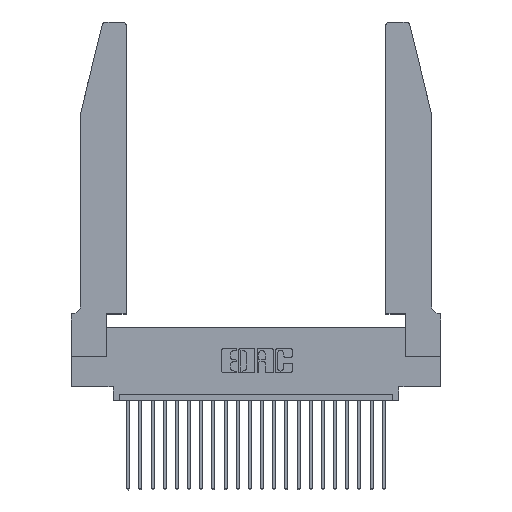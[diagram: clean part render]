
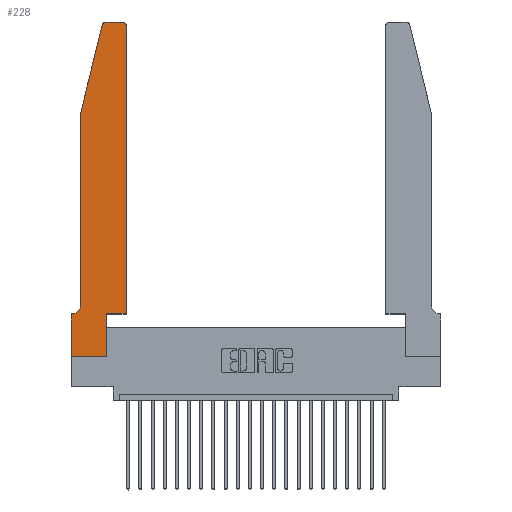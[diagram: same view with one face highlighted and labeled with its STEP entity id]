
A CAD part, top view. The second image highlights one B-rep face of the part: STEP entity #228.
In plain terms, the highlighted planar face has unit normal (0, 0, 1).
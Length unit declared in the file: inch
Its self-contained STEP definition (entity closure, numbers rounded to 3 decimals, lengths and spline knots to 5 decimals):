
#208 = DIRECTION ( 'NONE',  ( 0., -1., 0. ) ) ;
#228 = ADVANCED_FACE ( 'NONE', ( #15772 ), #24019, .T. ) ;
#949 = VECTOR ( 'NONE', #1038, 39.37008 ) ;
#1038 = DIRECTION ( 'NONE',  ( -0.239, -0.971, 0. ) ) ;
#1377 = VERTEX_POINT ( 'NONE', #22624 ) ;
#1398 = ORIENTED_EDGE ( 'NONE', *, *, #16703, .T. ) ;
#1642 = CARTESIAN_POINT ( 'NONE',  ( 0., 0.35, 0.37 ) ) ;
#1769 = VERTEX_POINT ( 'NONE', #23635 ) ;
#1843 = CARTESIAN_POINT ( 'NONE',  ( 0., 0.35, 0.37 ) ) ;
#1872 = ORIENTED_EDGE ( 'NONE', *, *, #16879, .T. ) ;
#2104 = LINE ( 'NONE', #21125, #12880 ) ;
#2142 = CARTESIAN_POINT ( 'NONE',  ( 0., 0., 0.37 ) ) ;
#2615 = VERTEX_POINT ( 'NONE', #24074 ) ;
#2848 = DIRECTION ( 'NONE',  ( 0., 0., -1. ) ) ;
#3400 = EDGE_CURVE ( 'NONE', #4514, #14230, #17943, .T. ) ;
#3630 = ORIENTED_EDGE ( 'NONE', *, *, #4726, .T. ) ;
#3846 = VERTEX_POINT ( 'NONE', #20107 ) ;
#3853 = EDGE_CURVE ( 'NONE', #1769, #8784, #18219, .T. ) ;
#4328 = DIRECTION ( 'NONE',  ( -1., 0., 0. ) ) ;
#4514 = VERTEX_POINT ( 'NONE', #21830 ) ;
#4726 = EDGE_CURVE ( 'NONE', #20221, #5148, #13159, .T. ) ;
#4738 = DIRECTION ( 'NONE',  ( -1., 0., 0. ) ) ;
#4908 = EDGE_CURVE ( 'NONE', #15444, #2615, #2104, .T. ) ;
#4972 = DIRECTION ( 'NONE',  ( 0., 1., 0. ) ) ;
#5030 = EDGE_CURVE ( 'NONE', #3846, #13183, #15221, .T. ) ;
#5148 = VERTEX_POINT ( 'NONE', #2142 ) ;
#5470 = EDGE_LOOP ( 'NONE', ( #20709, #20847, #14493, #20641, #1872, #21702, #3630, #16234, #9642, #24148, #1398, #8935 ) ) ;
#5584 = EDGE_CURVE ( 'NONE', #5148, #11150, #21610, .T. ) ;
#5921 = CARTESIAN_POINT ( 'NONE',  ( 0.0755, 0.35, 0.37 ) ) ;
#6894 = LINE ( 'NONE', #17451, #19441 ) ;
#7106 = VECTOR ( 'NONE', #10693, 39.37008 ) ;
#7161 = CIRCLE ( 'NONE', #9581, 0.07 ) ;
#8303 = CARTESIAN_POINT ( 'NONE',  ( 0.0755, 2., 0.37 ) ) ;
#8549 = CARTESIAN_POINT ( 'NONE',  ( 0.0755, 2., 0.37 ) ) ;
#8784 = VERTEX_POINT ( 'NONE', #10356 ) ;
#8935 = ORIENTED_EDGE ( 'NONE', *, *, #3853, .T. ) ;
#9190 = EDGE_CURVE ( 'NONE', #1377, #20221, #10885, .T. ) ;
#9581 = AXIS2_PLACEMENT_3D ( 'NONE', #14099, #2848, #4738 ) ;
#9642 = ORIENTED_EDGE ( 'NONE', *, *, #22647, .T. ) ;
#9996 = LINE ( 'NONE', #10611, #7106 ) ;
#10356 = CARTESIAN_POINT ( 'NONE',  ( 0.4205, 2.75, 0.37 ) ) ;
#10611 = CARTESIAN_POINT ( 'NONE',  ( 0.2865, 0.35, 0.37 ) ) ;
#10693 = DIRECTION ( 'NONE',  ( 0., 1., 0. ) ) ;
#10829 = VECTOR ( 'NONE', #208, 39.37008 ) ;
#10885 = LINE ( 'NONE', #5921, #21707 ) ;
#11150 = VERTEX_POINT ( 'NONE', #20236 ) ;
#11836 = DIRECTION ( 'NONE',  ( 0., -1., 0. ) ) ;
#12509 = DIRECTION ( 'NONE',  ( 1., 0., 0. ) ) ;
#12837 = DIRECTION ( 'NONE',  ( 1., 0., 0. ) ) ;
#12880 = VECTOR ( 'NONE', #11836, 39.37008 ) ;
#13157 = AXIS2_PLACEMENT_3D ( 'NONE', #13678, #17201, #17374 ) ;
#13159 = LINE ( 'NONE', #13223, #10829 ) ;
#13183 = VERTEX_POINT ( 'NONE', #17450 ) ;
#13223 = CARTESIAN_POINT ( 'NONE',  ( 0., 0., 0.37 ) ) ;
#13304 = AXIS2_PLACEMENT_3D ( 'NONE', #16375, #23688, #12509 ) ;
#13678 = CARTESIAN_POINT ( 'NONE',  ( 0.284, 2.72, 0.37 ) ) ;
#13995 = CARTESIAN_POINT ( 'NONE',  ( 0.4505, 0.35, 0.37 ) ) ;
#14099 = CARTESIAN_POINT ( 'NONE',  ( 0.0055, 0.42, 0.37 ) ) ;
#14230 = VERTEX_POINT ( 'NONE', #14533 ) ;
#14493 = ORIENTED_EDGE ( 'NONE', *, *, #19425, .T. ) ;
#14528 = EDGE_CURVE ( 'NONE', #8784, #3846, #6894, .T. ) ;
#14533 = CARTESIAN_POINT ( 'NONE',  ( 0.4505, 0.35, 0.37 ) ) ;
#14750 = LINE ( 'NONE', #19561, #15637 ) ;
#15221 = CIRCLE ( 'NONE', #13157, 0.03 ) ;
#15444 = VERTEX_POINT ( 'NONE', #8303 ) ;
#15637 = VECTOR ( 'NONE', #4972, 39.37008 ) ;
#15772 = FACE_OUTER_BOUND ( 'NONE', #5470, .T. ) ;
#16234 = ORIENTED_EDGE ( 'NONE', *, *, #5584, .T. ) ;
#16375 = CARTESIAN_POINT ( 'NONE',  ( 0.4205, 2.72, 0.37 ) ) ;
#16536 = CARTESIAN_POINT ( 'NONE',  ( 0., 0., 0.37 ) ) ;
#16703 = EDGE_CURVE ( 'NONE', #14230, #1769, #14750, .T. ) ;
#16879 = EDGE_CURVE ( 'NONE', #2615, #1377, #7161, .T. ) ;
#16889 = DIRECTION ( 'NONE',  ( 1., 0., 0. ) ) ;
#17201 = DIRECTION ( 'NONE',  ( 0., 0., 1. ) ) ;
#17374 = DIRECTION ( 'NONE',  ( 1., 0., 0. ) ) ;
#17450 = CARTESIAN_POINT ( 'NONE',  ( 0.25487, 2.72718, 0.37 ) ) ;
#17451 = CARTESIAN_POINT ( 'NONE',  ( 0.2605, 2.75, 0.37 ) ) ;
#17943 = LINE ( 'NONE', #13995, #21421 ) ;
#18219 = CIRCLE ( 'NONE', #13304, 0.03 ) ;
#18669 = LINE ( 'NONE', #8549, #949 ) ;
#19425 = EDGE_CURVE ( 'NONE', #13183, #15444, #18669, .T. ) ;
#19441 = VECTOR ( 'NONE', #4328, 39.37008 ) ;
#19561 = CARTESIAN_POINT ( 'NONE',  ( 0.4505, 0.35, 0.37 ) ) ;
#20107 = CARTESIAN_POINT ( 'NONE',  ( 0.284, 2.75, 0.37 ) ) ;
#20142 = VECTOR ( 'NONE', #22144, 39.37008 ) ;
#20221 = VERTEX_POINT ( 'NONE', #1642 ) ;
#20236 = CARTESIAN_POINT ( 'NONE',  ( 0.2865, 0., 0.37 ) ) ;
#20619 = AXIS2_PLACEMENT_3D ( 'NONE', #1843, #22287, #12837 ) ;
#20641 = ORIENTED_EDGE ( 'NONE', *, *, #4908, .T. ) ;
#20709 = ORIENTED_EDGE ( 'NONE', *, *, #14528, .T. ) ;
#20847 = ORIENTED_EDGE ( 'NONE', *, *, #5030, .T. ) ;
#21125 = CARTESIAN_POINT ( 'NONE',  ( 0.0755, 2., 0.37 ) ) ;
#21421 = VECTOR ( 'NONE', #16889, 39.37008 ) ;
#21610 = LINE ( 'NONE', #16536, #20142 ) ;
#21702 = ORIENTED_EDGE ( 'NONE', *, *, #9190, .T. ) ;
#21707 = VECTOR ( 'NONE', #22545, 39.37008 ) ;
#21830 = CARTESIAN_POINT ( 'NONE',  ( 0.2865, 0.35, 0.37 ) ) ;
#22144 = DIRECTION ( 'NONE',  ( 1., 0., 0. ) ) ;
#22287 = DIRECTION ( 'NONE',  ( 0., 0., 1. ) ) ;
#22545 = DIRECTION ( 'NONE',  ( -1., 0., 0. ) ) ;
#22624 = CARTESIAN_POINT ( 'NONE',  ( 0.0055, 0.35, 0.37 ) ) ;
#22647 = EDGE_CURVE ( 'NONE', #11150, #4514, #9996, .T. ) ;
#23635 = CARTESIAN_POINT ( 'NONE',  ( 0.4505, 2.72, 0.37 ) ) ;
#23688 = DIRECTION ( 'NONE',  ( 0., 0., 1. ) ) ;
#24019 = PLANE ( 'NONE',  #20619 ) ;
#24074 = CARTESIAN_POINT ( 'NONE',  ( 0.0755, 0.42, 0.37 ) ) ;
#24148 = ORIENTED_EDGE ( 'NONE', *, *, #3400, .T. ) ;
